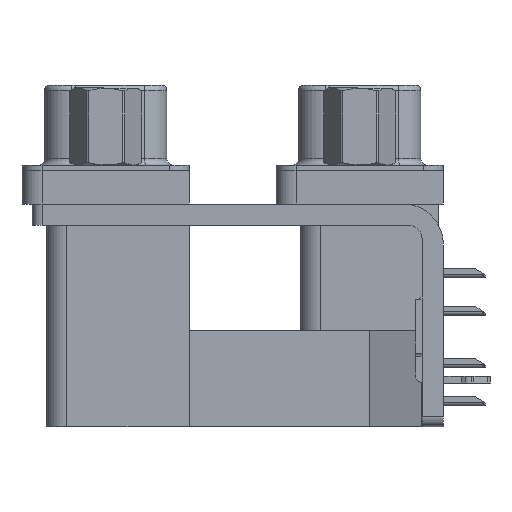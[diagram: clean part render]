
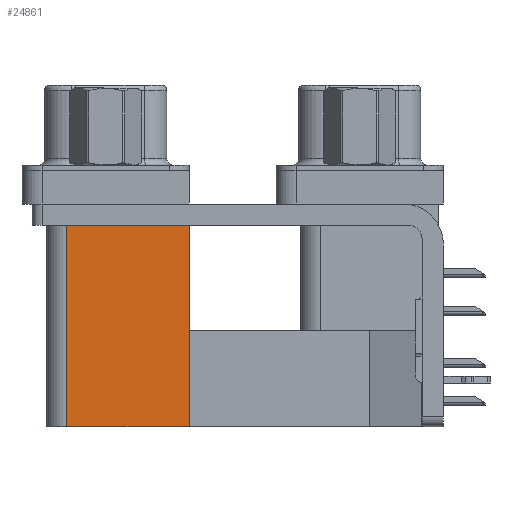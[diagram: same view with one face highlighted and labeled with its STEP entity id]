
A CAD part, left-side view. The second image highlights one B-rep face of the part: STEP entity #24861.
In plain terms, the highlighted planar face has unit normal (-1, 0, 0).
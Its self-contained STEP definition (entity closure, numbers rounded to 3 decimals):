
#515 = CARTESIAN_POINT ( 'NONE',  ( 3.79, 21.975, -19.2 ) ) ;
#950 = CARTESIAN_POINT ( 'NONE',  ( 3.79, 12.775, -2.5 ) ) ;
#1929 = EDGE_CURVE ( 'NONE', #16104, #23367, #7017, .T. ) ;
#2034 = DIRECTION ( 'NONE',  ( 0., 0., -1. ) ) ;
#2319 = ORIENTED_EDGE ( 'NONE', *, *, #8682, .T. ) ;
#2816 = EDGE_CURVE ( 'NONE', #23367, #21898, #23018, .T. ) ;
#3399 = DIRECTION ( 'NONE',  ( 0., 1., 0. ) ) ;
#4526 = DIRECTION ( 'NONE',  ( 1., 0., 0. ) ) ;
#5926 = LINE ( 'NONE', #25952, #26326 ) ;
#6986 = PLANE ( 'NONE',  #12470 ) ;
#7017 = LINE ( 'NONE', #14414, #19560 ) ;
#8682 = EDGE_CURVE ( 'NONE', #16104, #20925, #5926, .T. ) ;
#8969 = CARTESIAN_POINT ( 'NONE',  ( 3.79, 12.775, -2.5 ) ) ;
#9709 = CARTESIAN_POINT ( 'NONE',  ( 3.79, 21.975, -2.5 ) ) ;
#10564 = DIRECTION ( 'NONE',  ( 0., 0., 1. ) ) ;
#11082 = CARTESIAN_POINT ( 'NONE',  ( 3.79, 12.775, -19.2 ) ) ;
#11399 = ORIENTED_EDGE ( 'NONE', *, *, #21354, .T. ) ;
#12470 = AXIS2_PLACEMENT_3D ( 'NONE', #14056, #4526, #2034 ) ;
#14056 = CARTESIAN_POINT ( 'NONE',  ( 3.79, 12.775, -19.2 ) ) ;
#14414 = CARTESIAN_POINT ( 'NONE',  ( 3.79, 12.775, -19.2 ) ) ;
#16104 = VERTEX_POINT ( 'NONE', #11082 ) ;
#16158 = VECTOR ( 'NONE', #3399, 1000. ) ;
#17095 = ORIENTED_EDGE ( 'NONE', *, *, #2816, .F. ) ;
#19560 = VECTOR ( 'NONE', #26717, 1000. ) ;
#20925 = VERTEX_POINT ( 'NONE', #950 ) ;
#20996 = EDGE_LOOP ( 'NONE', ( #11399, #17095, #28695, #2319 ) ) ;
#21303 = VECTOR ( 'NONE', #10564, 1000. ) ;
#21354 = EDGE_CURVE ( 'NONE', #20925, #21898, #23744, .T. ) ;
#21898 = VERTEX_POINT ( 'NONE', #9709 ) ;
#23018 = LINE ( 'NONE', #515, #21303 ) ;
#23367 = VERTEX_POINT ( 'NONE', #28190 ) ;
#23744 = LINE ( 'NONE', #8969, #16158 ) ;
#24394 = FACE_OUTER_BOUND ( 'NONE', #20996, .T. ) ;
#24861 = ADVANCED_FACE ( 'NONE', ( #24394 ), #6986, .F. ) ;
#25952 = CARTESIAN_POINT ( 'NONE',  ( 3.79, 12.775, -19.2 ) ) ;
#26326 = VECTOR ( 'NONE', #28550, 1000. ) ;
#26717 = DIRECTION ( 'NONE',  ( 0., 1., 0. ) ) ;
#28190 = CARTESIAN_POINT ( 'NONE',  ( 3.79, 21.975, -19.2 ) ) ;
#28550 = DIRECTION ( 'NONE',  ( 0., 0., 1. ) ) ;
#28695 = ORIENTED_EDGE ( 'NONE', *, *, #1929, .F. ) ;
